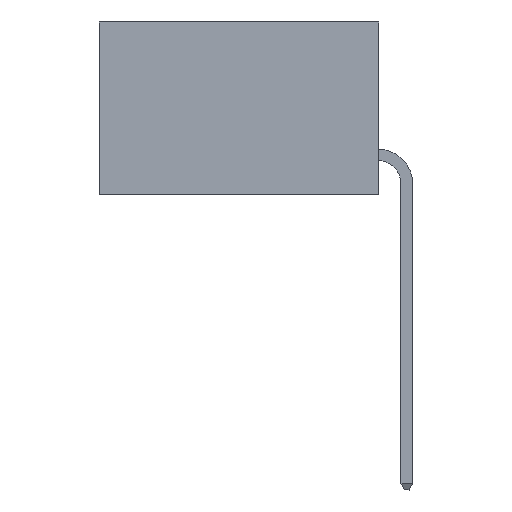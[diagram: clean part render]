
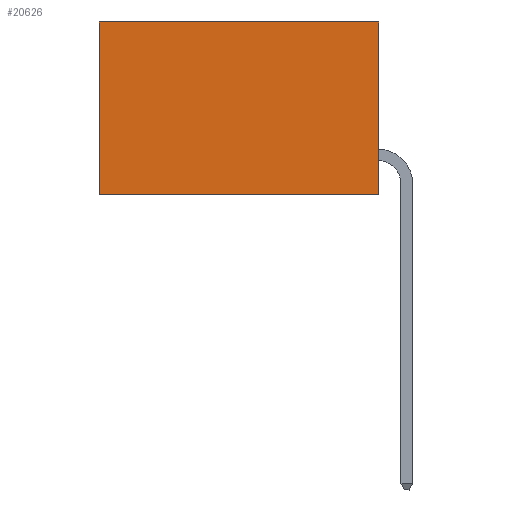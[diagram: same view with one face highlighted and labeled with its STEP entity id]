
A CAD part, left-side view. The second image highlights one B-rep face of the part: STEP entity #20626.
In plain terms, the highlighted planar face has unit normal (-1, 0, 0).
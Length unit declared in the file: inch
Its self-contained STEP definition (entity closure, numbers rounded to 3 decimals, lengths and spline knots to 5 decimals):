
#311 = DIRECTION ( 'NONE',  ( 1., 0., 0. ) ) ;
#1659 = VERTEX_POINT ( 'NONE', #3127 ) ;
#1775 = DIRECTION ( 'NONE',  ( 0., 0., -1. ) ) ;
#1781 = LINE ( 'NONE', #1893, #15304 ) ;
#1813 = VERTEX_POINT ( 'NONE', #1876 ) ;
#1876 = CARTESIAN_POINT ( 'NONE',  ( 0.2615, 0., 0. ) ) ;
#1893 = CARTESIAN_POINT ( 'NONE',  ( 0.2615, 0., 0. ) ) ;
#2078 = VECTOR ( 'NONE', #5788, 39.37008 ) ;
#2374 = VECTOR ( 'NONE', #3829, 39.37008 ) ;
#2445 = EDGE_CURVE ( 'NONE', #6109, #19403, #13291, .T. ) ;
#3127 = CARTESIAN_POINT ( 'NONE',  ( 0.2615, 0.6, 0. ) ) ;
#3708 = ORIENTED_EDGE ( 'NONE', *, *, #14403, .T. ) ;
#3829 = DIRECTION ( 'NONE',  ( 0., 0., -1. ) ) ;
#4211 = ORIENTED_EDGE ( 'NONE', *, *, #8085, .T. ) ;
#5402 = LINE ( 'NONE', #18166, #2374 ) ;
#5788 = DIRECTION ( 'NONE',  ( 0., 0., -1. ) ) ;
#5900 = CARTESIAN_POINT ( 'NONE',  ( 0.2615, 0., -0.37 ) ) ;
#6109 = VERTEX_POINT ( 'NONE', #5900 ) ;
#6508 = AXIS2_PLACEMENT_3D ( 'NONE', #19358, #311, #1775 ) ;
#6901 = DIRECTION ( 'NONE',  ( 0., 1., 0. ) ) ;
#7391 = CARTESIAN_POINT ( 'NONE',  ( 0.2615, 0.6, -0.37 ) ) ;
#7952 = ORIENTED_EDGE ( 'NONE', *, *, #15434, .F. ) ;
#8085 = EDGE_CURVE ( 'NONE', #1813, #1659, #1781, .T. ) ;
#8274 = DIRECTION ( 'NONE',  ( 0., 1., 0. ) ) ;
#10787 = ORIENTED_EDGE ( 'NONE', *, *, #2445, .F. ) ;
#11501 = CARTESIAN_POINT ( 'NONE',  ( 0.2615, 0., -0.37 ) ) ;
#13291 = LINE ( 'NONE', #11501, #18583 ) ;
#14403 = EDGE_CURVE ( 'NONE', #1659, #19403, #5402, .T. ) ;
#15304 = VECTOR ( 'NONE', #8274, 39.37008 ) ;
#15434 = EDGE_CURVE ( 'NONE', #1813, #6109, #18354, .T. ) ;
#16118 = PLANE ( 'NONE',  #6508 ) ;
#16331 = FACE_OUTER_BOUND ( 'NONE', #17284, .T. ) ;
#16885 = CARTESIAN_POINT ( 'NONE',  ( 0.2615, 0., -0.37 ) ) ;
#17284 = EDGE_LOOP ( 'NONE', ( #3708, #10787, #7952, #4211 ) ) ;
#18166 = CARTESIAN_POINT ( 'NONE',  ( 0.2615, 0.6, -0.37 ) ) ;
#18354 = LINE ( 'NONE', #16885, #2078 ) ;
#18583 = VECTOR ( 'NONE', #6901, 39.37008 ) ;
#19358 = CARTESIAN_POINT ( 'NONE',  ( 0.2615, 0., -0.37 ) ) ;
#19403 = VERTEX_POINT ( 'NONE', #7391 ) ;
#20626 = ADVANCED_FACE ( 'NONE', ( #16331 ), #16118, .F. ) ;
